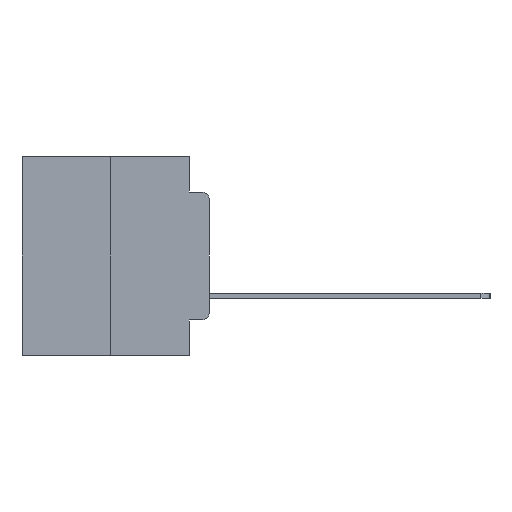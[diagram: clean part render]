
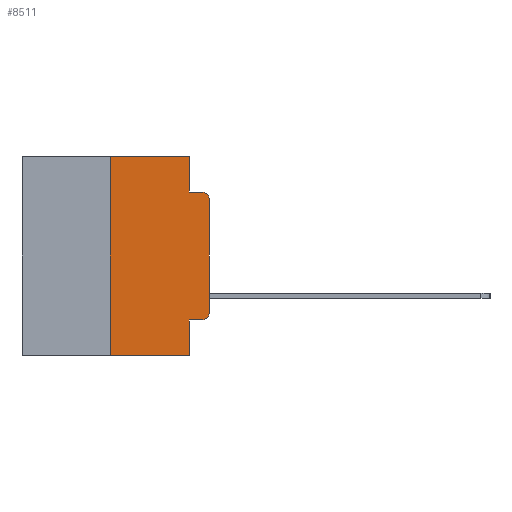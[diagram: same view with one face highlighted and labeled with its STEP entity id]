
A CAD part, left-side view. The second image highlights one B-rep face of the part: STEP entity #8511.
In plain terms, the highlighted planar face has unit normal (-1, 0, 0).
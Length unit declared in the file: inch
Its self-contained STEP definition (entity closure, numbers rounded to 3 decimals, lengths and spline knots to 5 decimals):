
#679 = CARTESIAN_POINT ( 'NONE',  ( 0., 0.051, -0.0885 ) ) ;
#825 = ORIENTED_EDGE ( 'NONE', *, *, #12277, .T. ) ;
#1342 = DIRECTION ( 'NONE',  ( 0., 0., -1. ) ) ;
#1495 = CIRCLE ( 'NONE', #21338, 0.02 ) ;
#2665 = LINE ( 'NONE', #23196, #24124 ) ;
#2698 = EDGE_CURVE ( 'NONE', #21263, #6822, #8153, .T. ) ;
#3914 = VERTEX_POINT ( 'NONE', #22654 ) ;
#3949 = DIRECTION ( 'NONE',  ( 0., 0., -1. ) ) ;
#4369 = VERTEX_POINT ( 'NONE', #18481 ) ;
#4682 = DIRECTION ( 'NONE',  ( 0., -1., 0. ) ) ;
#4978 = FACE_OUTER_BOUND ( 'NONE', #22624, .T. ) ;
#5073 = CARTESIAN_POINT ( 'NONE',  ( 0., 0.473, -0.5 ) ) ;
#5510 = CARTESIAN_POINT ( 'NONE',  ( 0., 0.051, -0.4115 ) ) ;
#6231 = DIRECTION ( 'NONE',  ( -1., 0., 0. ) ) ;
#6690 = EDGE_CURVE ( 'NONE', #4369, #14609, #2665, .T. ) ;
#6822 = VERTEX_POINT ( 'NONE', #679 ) ;
#7384 = ORIENTED_EDGE ( 'NONE', *, *, #22480, .T. ) ;
#7395 = VERTEX_POINT ( 'NONE', #21737 ) ;
#7658 = EDGE_CURVE ( 'NONE', #7395, #8310, #14917, .T. ) ;
#8153 = LINE ( 'NONE', #22341, #18420 ) ;
#8310 = VERTEX_POINT ( 'NONE', #8483 ) ;
#8319 = CARTESIAN_POINT ( 'NONE',  ( 0., 0., 0. ) ) ;
#8483 = CARTESIAN_POINT ( 'NONE',  ( 0., 0.02, -0.0885 ) ) ;
#8511 = ADVANCED_FACE ( 'NONE', ( #4978 ), #9048, .F. ) ;
#8527 = VERTEX_POINT ( 'NONE', #17295 ) ;
#8812 = LINE ( 'NONE', #8319, #19051 ) ;
#8958 = CARTESIAN_POINT ( 'NONE',  ( 0., 0.051, -0.0885 ) ) ;
#9048 = PLANE ( 'NONE',  #25932 ) ;
#9470 = CARTESIAN_POINT ( 'NONE',  ( 0., 0.25, 0. ) ) ;
#9642 = CARTESIAN_POINT ( 'NONE',  ( 0., 0.051, 0. ) ) ;
#10583 = CARTESIAN_POINT ( 'NONE',  ( 0., 0.051, -0.5 ) ) ;
#10868 = CARTESIAN_POINT ( 'NONE',  ( 0., 0.473, 0. ) ) ;
#11092 = DIRECTION ( 'NONE',  ( 0., 0., -1. ) ) ;
#11980 = VERTEX_POINT ( 'NONE', #9470 ) ;
#12010 = LINE ( 'NONE', #8958, #16728 ) ;
#12201 = DIRECTION ( 'NONE',  ( 0., 0., 1. ) ) ;
#12277 = EDGE_CURVE ( 'NONE', #8527, #7395, #8812, .T. ) ;
#13248 = DIRECTION ( 'NONE',  ( 0., 0., -1. ) ) ;
#13758 = EDGE_CURVE ( 'NONE', #3914, #8527, #1495, .T. ) ;
#14195 = DIRECTION ( 'NONE',  ( -1., 0., 0. ) ) ;
#14609 = VERTEX_POINT ( 'NONE', #10583 ) ;
#14743 = LINE ( 'NONE', #26346, #20097 ) ;
#14805 = ORIENTED_EDGE ( 'NONE', *, *, #6690, .F. ) ;
#14917 = CIRCLE ( 'NONE', #19356, 0.02 ) ;
#15511 = ORIENTED_EDGE ( 'NONE', *, *, #2698, .F. ) ;
#15527 = LINE ( 'NONE', #5073, #20248 ) ;
#15932 = DIRECTION ( 'NONE',  ( 0., -1., 0. ) ) ;
#16728 = VECTOR ( 'NONE', #4682, 39.37008 ) ;
#16791 = EDGE_CURVE ( 'NONE', #6822, #8310, #12010, .T. ) ;
#17295 = CARTESIAN_POINT ( 'NONE',  ( 0., 0., -0.3915 ) ) ;
#17729 = ORIENTED_EDGE ( 'NONE', *, *, #13758, .T. ) ;
#18388 = VECTOR ( 'NONE', #25086, 39.37008 ) ;
#18420 = VECTOR ( 'NONE', #3949, 39.37008 ) ;
#18481 = CARTESIAN_POINT ( 'NONE',  ( 0., 0.051, -0.4115 ) ) ;
#18637 = CARTESIAN_POINT ( 'NONE',  ( 0., 0.02, -0.1085 ) ) ;
#19051 = VECTOR ( 'NONE', #24638, 39.37008 ) ;
#19356 = AXIS2_PLACEMENT_3D ( 'NONE', #18637, #6231, #20668 ) ;
#19916 = ORIENTED_EDGE ( 'NONE', *, *, #23392, .T. ) ;
#20097 = VECTOR ( 'NONE', #12201, 39.37008 ) ;
#20248 = VECTOR ( 'NONE', #25550, 39.37008 ) ;
#20668 = DIRECTION ( 'NONE',  ( 0., 0., -1. ) ) ;
#20863 = ORIENTED_EDGE ( 'NONE', *, *, #26025, .F. ) ;
#20924 = LINE ( 'NONE', #5510, #25641 ) ;
#21263 = VERTEX_POINT ( 'NONE', #9642 ) ;
#21338 = AXIS2_PLACEMENT_3D ( 'NONE', #26229, #14195, #1342 ) ;
#21737 = CARTESIAN_POINT ( 'NONE',  ( 0., 0., -0.1085 ) ) ;
#22125 = ORIENTED_EDGE ( 'NONE', *, *, #7658, .T. ) ;
#22341 = CARTESIAN_POINT ( 'NONE',  ( 0., 0.051, 0. ) ) ;
#22480 = EDGE_CURVE ( 'NONE', #4369, #3914, #20924, .T. ) ;
#22545 = EDGE_CURVE ( 'NONE', #11980, #21263, #23762, .T. ) ;
#22624 = EDGE_LOOP ( 'NONE', ( #825, #22125, #26787, #15511, #23057, #20863, #19916, #14805, #7384, #17729 ) ) ;
#22654 = CARTESIAN_POINT ( 'NONE',  ( 0., 0.02, -0.4115 ) ) ;
#23057 = ORIENTED_EDGE ( 'NONE', *, *, #22545, .F. ) ;
#23196 = CARTESIAN_POINT ( 'NONE',  ( 0., 0.051, 0. ) ) ;
#23236 = VERTEX_POINT ( 'NONE', #25142 ) ;
#23292 = CARTESIAN_POINT ( 'NONE',  ( 0., 0.473, 0. ) ) ;
#23392 = EDGE_CURVE ( 'NONE', #23236, #14609, #15527, .T. ) ;
#23762 = LINE ( 'NONE', #10868, #18388 ) ;
#24124 = VECTOR ( 'NONE', #11092, 39.37008 ) ;
#24638 = DIRECTION ( 'NONE',  ( 0., 0., 1. ) ) ;
#25086 = DIRECTION ( 'NONE',  ( 0., -1., 0. ) ) ;
#25142 = CARTESIAN_POINT ( 'NONE',  ( 0., 0.25, -0.5 ) ) ;
#25302 = DIRECTION ( 'NONE',  ( 1., 0., 0. ) ) ;
#25550 = DIRECTION ( 'NONE',  ( 0., -1., 0. ) ) ;
#25641 = VECTOR ( 'NONE', #15932, 39.37008 ) ;
#25932 = AXIS2_PLACEMENT_3D ( 'NONE', #23292, #25302, #13248 ) ;
#26025 = EDGE_CURVE ( 'NONE', #23236, #11980, #14743, .T. ) ;
#26229 = CARTESIAN_POINT ( 'NONE',  ( 0., 0.02, -0.3915 ) ) ;
#26346 = CARTESIAN_POINT ( 'NONE',  ( 0., 0.25, 0. ) ) ;
#26787 = ORIENTED_EDGE ( 'NONE', *, *, #16791, .F. ) ;
